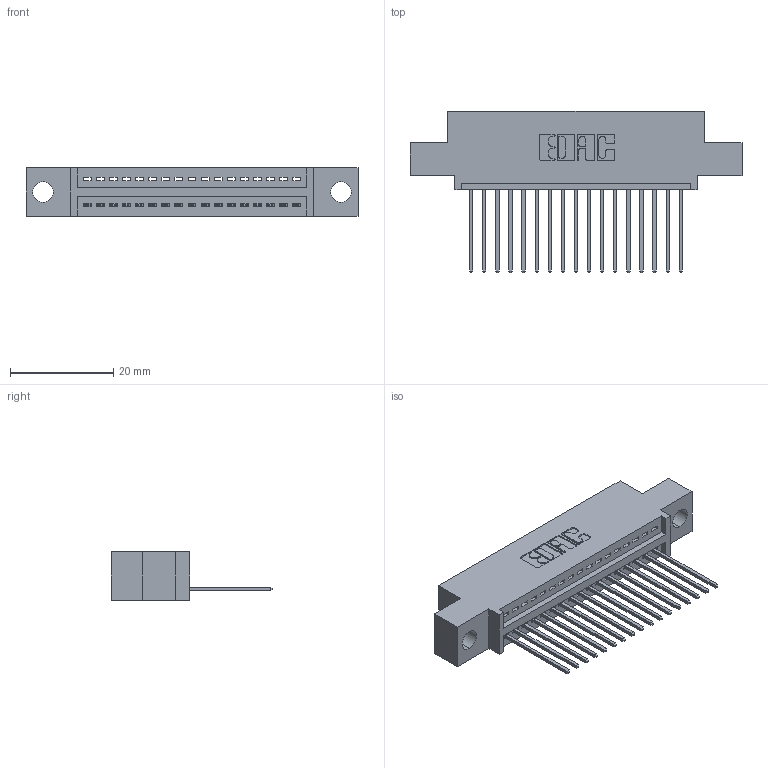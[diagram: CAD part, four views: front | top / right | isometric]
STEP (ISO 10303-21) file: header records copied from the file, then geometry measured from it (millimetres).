
FILE_DESCRIPTION (( 'STEP AP203' ), '1' );
FILE_NAME ('395-017-542-404.STEP', '2021-05-31T14:24:56', ( '' ), ( '' ), 'SwSTEP 2.0', 'SolidWorks 2020', '' );
FILE_SCHEMA (( 'CONFIG_CONTROL_DESIGN' ));
Length unit declared in the file: inch
Products named in the file (3): 345-292-001_345-293-142; 345 Part_0.110 Offset - 0.156 Dia-TI; 395-017-542-404
Assembly tree (18 placements, depth 2):
  395-017-542-404
    345 Part_0.110 Offset - 0.156 Dia-TI
    345-292-001_345-293-142  x17
Bounding box: 64.39 x 31.29 x 9.4 mm (x, y, z)
Volume: 5769.4 mm3; surface area: 7490.9 mm2
Topology: 18 solids, 18 shells, 1130 faces, 3381 edges, 2230 vertices
Faces by surface type: plane 778, cylinder 352
Entity records: 16729 total; most frequent: CARTESIAN_POINT 2909, ORIENTED_EDGE 2858, DIRECTION 2575, EDGE_CURVE 1429, LINE 1229, VECTOR 1229, VERTEX_POINT 950, AXIS2_PLACEMENT_3D 673
